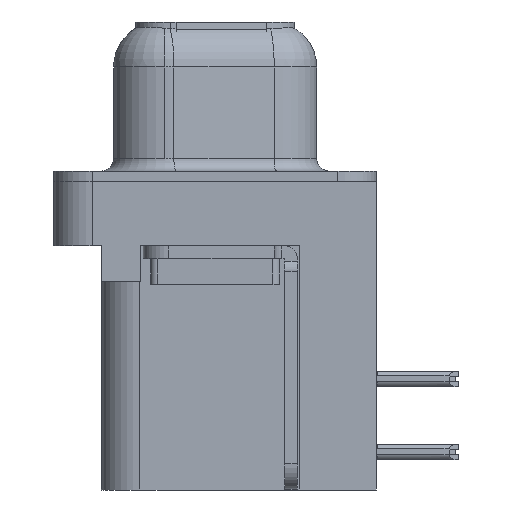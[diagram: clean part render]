
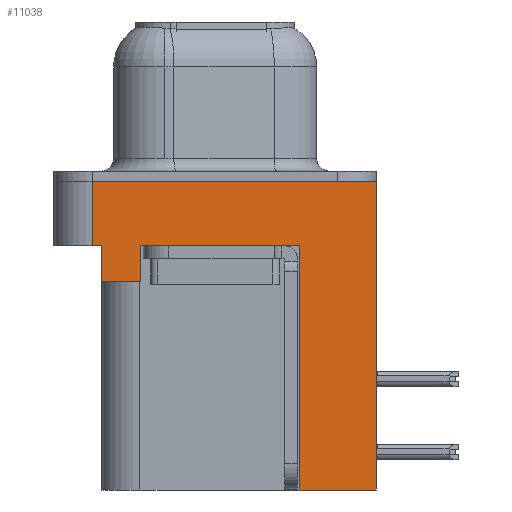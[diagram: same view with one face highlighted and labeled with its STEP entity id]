
A CAD part, left-side view. The second image highlights one B-rep face of the part: STEP entity #11038.
In plain terms, the highlighted planar face has unit normal (-1, 0, 0).
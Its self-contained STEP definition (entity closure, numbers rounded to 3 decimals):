
#12 = CARTESIAN_POINT ( 'NONE',  ( -2.935, -3.295, -12. ) ) ;
#495 = CARTESIAN_POINT ( 'NONE',  ( -2.935, 2.895, -3.9 ) ) ;
#645 = CARTESIAN_POINT ( 'NONE',  ( -2.935, -6.275, 0. ) ) ;
#673 = VERTEX_POINT ( 'NONE', #2326 ) ;
#722 = CARTESIAN_POINT ( 'NONE',  ( -2.935, 4.425, -3.9 ) ) ;
#878 = VECTOR ( 'NONE', #12529, 1000. ) ;
#1963 = EDGE_CURVE ( 'NONE', #25423, #2263, #14043, .T. ) ;
#2243 = EDGE_CURVE ( 'NONE', #18608, #16744, #20451, .T. ) ;
#2263 = VERTEX_POINT ( 'NONE', #722 ) ;
#2267 = CARTESIAN_POINT ( 'NONE',  ( -2.935, -6.275, 0. ) ) ;
#2326 = CARTESIAN_POINT ( 'NONE',  ( -2.935, -6.275, -12. ) ) ;
#3948 = VECTOR ( 'NONE', #8248, 1000. ) ;
#4251 = VERTEX_POINT ( 'NONE', #12 ) ;
#4281 = CARTESIAN_POINT ( 'NONE',  ( -2.935, 4.425, -3.9 ) ) ;
#4349 = CARTESIAN_POINT ( 'NONE',  ( -2.935, 2.895, -2.5 ) ) ;
#4354 = EDGE_CURVE ( 'NONE', #673, #16744, #13568, .T. ) ;
#4366 = DIRECTION ( 'NONE',  ( 0., 0., 1. ) ) ;
#4807 = ORIENTED_EDGE ( 'NONE', *, *, #9378, .F. ) ;
#4836 = VERTEX_POINT ( 'NONE', #5634 ) ;
#4848 = PLANE ( 'NONE',  #21239 ) ;
#5070 = CARTESIAN_POINT ( 'NONE',  ( -2.935, 4.425, -3.9 ) ) ;
#5149 = EDGE_CURVE ( 'NONE', #4251, #4836, #9081, .T. ) ;
#5634 = CARTESIAN_POINT ( 'NONE',  ( -2.935, -3.295, -2.5 ) ) ;
#5865 = ORIENTED_EDGE ( 'NONE', *, *, #16775, .T. ) ;
#6129 = LINE ( 'NONE', #13261, #10283 ) ;
#6338 = DIRECTION ( 'NONE',  ( 0., -1., 0. ) ) ;
#6827 = DIRECTION ( 'NONE',  ( 0., 0., 1. ) ) ;
#7694 = CARTESIAN_POINT ( 'NONE',  ( -2.935, -3.295, -12. ) ) ;
#7873 = DIRECTION ( 'NONE',  ( 0., 0., 1. ) ) ;
#8248 = DIRECTION ( 'NONE',  ( 0., 0., 1. ) ) ;
#8325 = VECTOR ( 'NONE', #18244, 1000. ) ;
#9059 = EDGE_CURVE ( 'NONE', #2263, #12415, #17834, .T. ) ;
#9081 = LINE ( 'NONE', #24189, #26140 ) ;
#9378 = EDGE_CURVE ( 'NONE', #23639, #18608, #18757, .T. ) ;
#10018 = ORIENTED_EDGE ( 'NONE', *, *, #9059, .F. ) ;
#10159 = VECTOR ( 'NONE', #12989, 1000. ) ;
#10283 = VECTOR ( 'NONE', #25908, 1000. ) ;
#10615 = CARTESIAN_POINT ( 'NONE',  ( -2.935, -6.275, -2.5 ) ) ;
#10812 = ORIENTED_EDGE ( 'NONE', *, *, #12789, .F. ) ;
#11030 = VECTOR ( 'NONE', #4366, 1000. ) ;
#11038 = ADVANCED_FACE ( 'NONE', ( #14540 ), #4848, .T. ) ;
#12114 = EDGE_CURVE ( 'NONE', #25423, #25129, #14454, .T. ) ;
#12415 = VERTEX_POINT ( 'NONE', #16270 ) ;
#12447 = CARTESIAN_POINT ( 'NONE',  ( -2.935, -6.275, -2.5 ) ) ;
#12529 = DIRECTION ( 'NONE',  ( 0., -1., 0. ) ) ;
#12789 = EDGE_CURVE ( 'NONE', #673, #4251, #14128, .T. ) ;
#12989 = DIRECTION ( 'NONE',  ( 0., 1., 0. ) ) ;
#13261 = CARTESIAN_POINT ( 'NONE',  ( -2.935, -6.275, -2.5 ) ) ;
#13568 = LINE ( 'NONE', #10615, #3948 ) ;
#14043 = LINE ( 'NONE', #5070, #10159 ) ;
#14128 = LINE ( 'NONE', #7694, #8325 ) ;
#14193 = ORIENTED_EDGE ( 'NONE', *, *, #4354, .T. ) ;
#14454 = LINE ( 'NONE', #21646, #16084 ) ;
#14540 = FACE_OUTER_BOUND ( 'NONE', #15804, .T. ) ;
#15283 = DIRECTION ( 'NONE',  ( 0., 0., 1. ) ) ;
#15804 = EDGE_LOOP ( 'NONE', ( #24127, #4807, #16891, #10018, #15939, #17991, #5865, #17004, #10812, #14193 ) ) ;
#15939 = ORIENTED_EDGE ( 'NONE', *, *, #1963, .F. ) ;
#16040 = CARTESIAN_POINT ( 'NONE',  ( -2.935, 4.775, -2.5 ) ) ;
#16084 = VECTOR ( 'NONE', #15283, 1000. ) ;
#16270 = CARTESIAN_POINT ( 'NONE',  ( -2.935, 4.425, -2.5 ) ) ;
#16744 = VERTEX_POINT ( 'NONE', #645 ) ;
#16775 = EDGE_CURVE ( 'NONE', #25129, #4836, #6129, .T. ) ;
#16891 = ORIENTED_EDGE ( 'NONE', *, *, #19505, .T. ) ;
#17004 = ORIENTED_EDGE ( 'NONE', *, *, #5149, .F. ) ;
#17834 = LINE ( 'NONE', #4281, #11030 ) ;
#17991 = ORIENTED_EDGE ( 'NONE', *, *, #12114, .T. ) ;
#18244 = DIRECTION ( 'NONE',  ( 0., 1., 0. ) ) ;
#18608 = VERTEX_POINT ( 'NONE', #21232 ) ;
#18757 = LINE ( 'NONE', #20281, #24503 ) ;
#19505 = EDGE_CURVE ( 'NONE', #23639, #12415, #20771, .T. ) ;
#20258 = DIRECTION ( 'NONE',  ( 0., 0., 1. ) ) ;
#20281 = CARTESIAN_POINT ( 'NONE',  ( -2.935, 4.775, -2.5 ) ) ;
#20451 = LINE ( 'NONE', #2267, #21363 ) ;
#20771 = LINE ( 'NONE', #12447, #878 ) ;
#21022 = CARTESIAN_POINT ( 'NONE',  ( -2.935, -6.275, -2.5 ) ) ;
#21232 = CARTESIAN_POINT ( 'NONE',  ( -2.935, 4.775, 0. ) ) ;
#21239 = AXIS2_PLACEMENT_3D ( 'NONE', #21022, #23037, #6827 ) ;
#21363 = VECTOR ( 'NONE', #6338, 1000. ) ;
#21646 = CARTESIAN_POINT ( 'NONE',  ( -2.935, 2.895, -3.9 ) ) ;
#23037 = DIRECTION ( 'NONE',  ( -1., 0., 0. ) ) ;
#23639 = VERTEX_POINT ( 'NONE', #16040 ) ;
#24127 = ORIENTED_EDGE ( 'NONE', *, *, #2243, .F. ) ;
#24189 = CARTESIAN_POINT ( 'NONE',  ( -2.935, -3.295, -12. ) ) ;
#24503 = VECTOR ( 'NONE', #7873, 1000. ) ;
#25129 = VERTEX_POINT ( 'NONE', #4349 ) ;
#25423 = VERTEX_POINT ( 'NONE', #495 ) ;
#25908 = DIRECTION ( 'NONE',  ( 0., -1., 0. ) ) ;
#26140 = VECTOR ( 'NONE', #20258, 1000. ) ;
